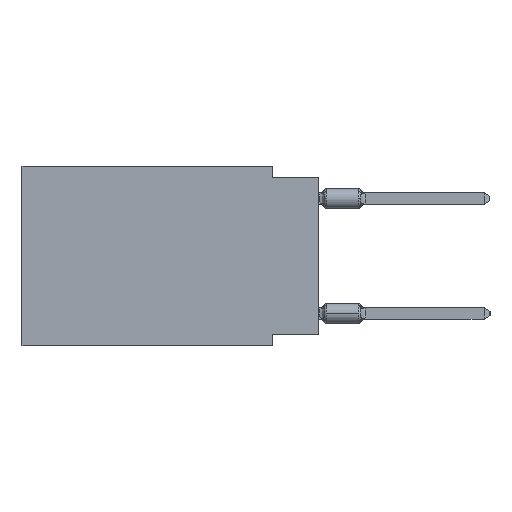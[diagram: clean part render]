
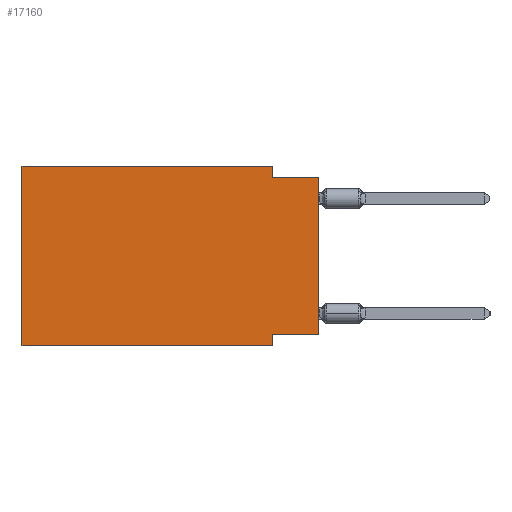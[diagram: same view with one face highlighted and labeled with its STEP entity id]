
A CAD part, left-side view. The second image highlights one B-rep face of the part: STEP entity #17160.
In plain terms, the highlighted planar face has unit normal (-1, 0, 0).
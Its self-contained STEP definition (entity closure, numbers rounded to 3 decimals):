
#937 = DIRECTION ( 'NONE',  ( 0., -1., 0. ) ) ;
#1704 = EDGE_CURVE ( 'NONE', #15145, #53039, #21311, .T. ) ;
#2260 = DIRECTION ( 'NONE',  ( 0., 0., 1. ) ) ;
#2423 = EDGE_CURVE ( 'NONE', #3360, #15145, #41525, .T. ) ;
#3221 = CARTESIAN_POINT ( 'NONE',  ( 0., 16.383, 0. ) ) ;
#3360 = VERTEX_POINT ( 'NONE', #18264 ) ;
#4368 = CARTESIAN_POINT ( 'NONE',  ( 0., 2.54, 0. ) ) ;
#4893 = CARTESIAN_POINT ( 'NONE',  ( 0., 0., -0.635 ) ) ;
#7358 = LINE ( 'NONE', #23933, #42757 ) ;
#8450 = DIRECTION ( 'NONE',  ( 0., 0., -1. ) ) ;
#9134 = EDGE_CURVE ( 'NONE', #38816, #25222, #18368, .T. ) ;
#9848 = VECTOR ( 'NONE', #28443, 1000. ) ;
#11445 = EDGE_CURVE ( 'NONE', #18696, #36574, #7358, .T. ) ;
#11691 = DIRECTION ( 'NONE',  ( 0., 1., 0. ) ) ;
#11721 = ORIENTED_EDGE ( 'NONE', *, *, #27876, .F. ) ;
#11870 = LINE ( 'NONE', #22096, #9848 ) ;
#13618 = ORIENTED_EDGE ( 'NONE', *, *, #25482, .F. ) ;
#13838 = VECTOR ( 'NONE', #937, 1000. ) ;
#14220 = CARTESIAN_POINT ( 'NONE',  ( 0., 2.54, -9.271 ) ) ;
#15145 = VERTEX_POINT ( 'NONE', #29056 ) ;
#15565 = CARTESIAN_POINT ( 'NONE',  ( 0., 0., 0. ) ) ;
#15735 = CARTESIAN_POINT ( 'NONE',  ( 0., 0., -9.271 ) ) ;
#17127 = CARTESIAN_POINT ( 'NONE',  ( 0., 2.54, -9.906 ) ) ;
#17160 = ADVANCED_FACE ( 'NONE', ( #36932 ), #32878, .F. ) ;
#18264 = CARTESIAN_POINT ( 'NONE',  ( 0., 2.54, 0. ) ) ;
#18368 = LINE ( 'NONE', #22979, #42698 ) ;
#18696 = VERTEX_POINT ( 'NONE', #15735 ) ;
#19153 = EDGE_LOOP ( 'NONE', ( #49654, #30684, #51948, #11721, #29885, #24054, #13618, #28279 ) ) ;
#20916 = DIRECTION ( 'NONE',  ( 0., 0., -1. ) ) ;
#21311 = LINE ( 'NONE', #33783, #13838 ) ;
#21907 = CARTESIAN_POINT ( 'NONE',  ( 0., 2.54, -9.906 ) ) ;
#22096 = CARTESIAN_POINT ( 'NONE',  ( 0., 16.383, -9.906 ) ) ;
#22714 = DIRECTION ( 'NONE',  ( 0., 0., -1. ) ) ;
#22979 = CARTESIAN_POINT ( 'NONE',  ( 0., 16.383, 0. ) ) ;
#23436 = EDGE_CURVE ( 'NONE', #18696, #53039, #44280, .T. ) ;
#23933 = CARTESIAN_POINT ( 'NONE',  ( 0., 0., -9.271 ) ) ;
#24054 = ORIENTED_EDGE ( 'NONE', *, *, #50759, .T. ) ;
#25222 = VERTEX_POINT ( 'NONE', #3221 ) ;
#25482 = EDGE_CURVE ( 'NONE', #36574, #29795, #51433, .T. ) ;
#27783 = VECTOR ( 'NONE', #2260, 1000. ) ;
#27860 = CARTESIAN_POINT ( 'NONE',  ( 0., 16.383, -9.906 ) ) ;
#27876 = EDGE_CURVE ( 'NONE', #25222, #3360, #39928, .T. ) ;
#28275 = CARTESIAN_POINT ( 'NONE',  ( 0., 16.383, 0. ) ) ;
#28279 = ORIENTED_EDGE ( 'NONE', *, *, #11445, .F. ) ;
#28443 = DIRECTION ( 'NONE',  ( 0., -1., 0. ) ) ;
#29056 = CARTESIAN_POINT ( 'NONE',  ( 0., 2.54, -0.635 ) ) ;
#29079 = CARTESIAN_POINT ( 'NONE',  ( 0., 16.383, 0. ) ) ;
#29795 = VERTEX_POINT ( 'NONE', #17127 ) ;
#29885 = ORIENTED_EDGE ( 'NONE', *, *, #9134, .F. ) ;
#30684 = ORIENTED_EDGE ( 'NONE', *, *, #1704, .F. ) ;
#31377 = DIRECTION ( 'NONE',  ( 0., 0., 1. ) ) ;
#31857 = AXIS2_PLACEMENT_3D ( 'NONE', #29079, #45590, #8450 ) ;
#32878 = PLANE ( 'NONE',  #31857 ) ;
#33783 = CARTESIAN_POINT ( 'NONE',  ( 0., 0., -0.635 ) ) ;
#34746 = VECTOR ( 'NONE', #20916, 1000. ) ;
#35723 = VECTOR ( 'NONE', #22714, 1000. ) ;
#36574 = VERTEX_POINT ( 'NONE', #14220 ) ;
#36932 = FACE_OUTER_BOUND ( 'NONE', #19153, .T. ) ;
#38816 = VERTEX_POINT ( 'NONE', #27860 ) ;
#39928 = LINE ( 'NONE', #28275, #53080 ) ;
#41525 = LINE ( 'NONE', #4368, #34746 ) ;
#42698 = VECTOR ( 'NONE', #31377, 1000. ) ;
#42757 = VECTOR ( 'NONE', #11691, 1000. ) ;
#44280 = LINE ( 'NONE', #15565, #27783 ) ;
#45590 = DIRECTION ( 'NONE',  ( 1., 0., 0. ) ) ;
#49654 = ORIENTED_EDGE ( 'NONE', *, *, #23436, .T. ) ;
#50759 = EDGE_CURVE ( 'NONE', #38816, #29795, #11870, .T. ) ;
#51433 = LINE ( 'NONE', #21907, #35723 ) ;
#51868 = DIRECTION ( 'NONE',  ( 0., -1., 0. ) ) ;
#51948 = ORIENTED_EDGE ( 'NONE', *, *, #2423, .F. ) ;
#53039 = VERTEX_POINT ( 'NONE', #4893 ) ;
#53080 = VECTOR ( 'NONE', #51868, 1000. ) ;
